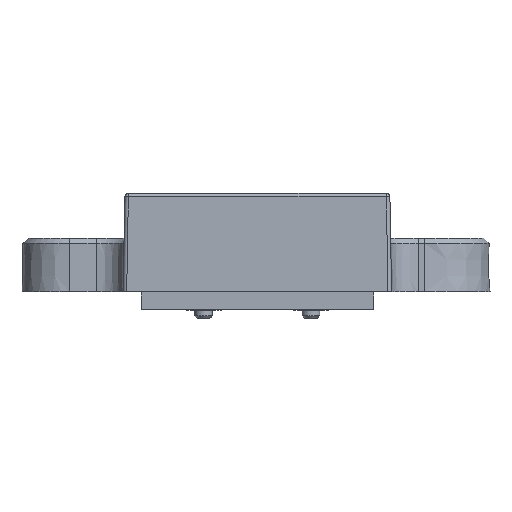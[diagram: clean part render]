
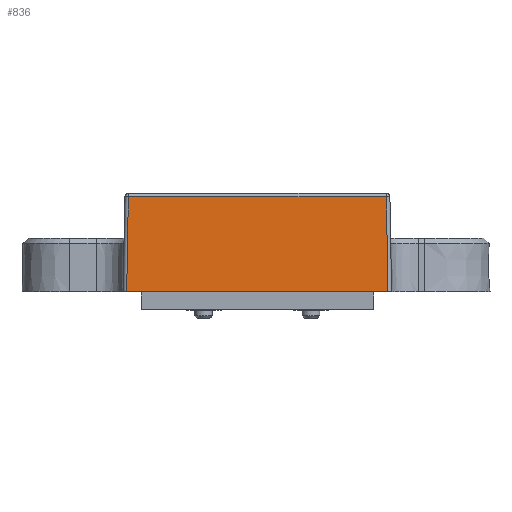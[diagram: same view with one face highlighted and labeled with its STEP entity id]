
A CAD part, left-side view. The second image highlights one B-rep face of the part: STEP entity #836.
In plain terms, the highlighted planar face has unit normal (-1, 0, 0.018).
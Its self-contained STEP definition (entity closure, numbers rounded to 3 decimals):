
#836 = ADVANCED_FACE ( 'NONE', ( #12670 ), #2323, .F. ) ;
#1189 = DIRECTION ( 'NONE',  ( 0., -1., 0. ) ) ;
#1268 = EDGE_CURVE ( 'NONE', #3279, #5187, #12795, .T. ) ;
#1419 = CARTESIAN_POINT ( 'NONE',  ( -17., 7.3, -5.5 ) ) ;
#1677 = EDGE_CURVE ( 'NONE', #14530, #8210, #9608, .T. ) ;
#1957 = EDGE_CURVE ( 'NONE', #8210, #3279, #11774, .T. ) ;
#2185 = CARTESIAN_POINT ( 'NONE',  ( -16.907, -7.207, -0.197 ) ) ;
#2323 = PLANE ( 'NONE',  #6677 ) ;
#2453 = CARTESIAN_POINT ( 'NONE',  ( -17., -7.3, -5.5 ) ) ;
#3279 = VERTEX_POINT ( 'NONE', #13879 ) ;
#3854 = DIRECTION ( 'NONE',  ( -0.017, 0.017, -1. ) ) ;
#5187 = VERTEX_POINT ( 'NONE', #9786 ) ;
#5796 = CARTESIAN_POINT ( 'NONE',  ( -16.907, 7.207, -0.197 ) ) ;
#6032 = DIRECTION ( 'NONE',  ( 0., -1., 0. ) ) ;
#6677 = AXIS2_PLACEMENT_3D ( 'NONE', #6950, #11542, #1189 ) ;
#6803 = DIRECTION ( 'NONE',  ( 0., 1., 0. ) ) ;
#6950 = CARTESIAN_POINT ( 'NONE',  ( -16.954, 0., -2.848 ) ) ;
#7079 = DIRECTION ( 'NONE',  ( 0.017, 0.017, 1. ) ) ;
#7343 = CARTESIAN_POINT ( 'NONE',  ( -17., 7.3, -5.5 ) ) ;
#8210 = VERTEX_POINT ( 'NONE', #7343 ) ;
#8333 = EDGE_CURVE ( 'NONE', #5187, #14530, #12531, .T. ) ;
#9608 = LINE ( 'NONE', #14212, #10751 ) ;
#9786 = CARTESIAN_POINT ( 'NONE',  ( -16.907, -7.207, -0.197 ) ) ;
#10751 = VECTOR ( 'NONE', #3854, 1000. ) ;
#11542 = DIRECTION ( 'NONE',  ( 1., 0., -0.017 ) ) ;
#11774 = LINE ( 'NONE', #1419, #14075 ) ;
#12416 = ORIENTED_EDGE ( 'NONE', *, *, #1957, .T. ) ;
#12531 = LINE ( 'NONE', #2185, #13412 ) ;
#12670 = FACE_OUTER_BOUND ( 'NONE', #13155, .T. ) ;
#12795 = LINE ( 'NONE', #2453, #13021 ) ;
#13021 = VECTOR ( 'NONE', #7079, 1000. ) ;
#13107 = ORIENTED_EDGE ( 'NONE', *, *, #8333, .T. ) ;
#13155 = EDGE_LOOP ( 'NONE', ( #13107, #14629, #12416, #13996 ) ) ;
#13412 = VECTOR ( 'NONE', #6803, 1000. ) ;
#13879 = CARTESIAN_POINT ( 'NONE',  ( -17., -7.3, -5.5 ) ) ;
#13996 = ORIENTED_EDGE ( 'NONE', *, *, #1268, .T. ) ;
#14075 = VECTOR ( 'NONE', #6032, 1000. ) ;
#14212 = CARTESIAN_POINT ( 'NONE',  ( -16.907, 7.207, -0.197 ) ) ;
#14530 = VERTEX_POINT ( 'NONE', #5796 ) ;
#14629 = ORIENTED_EDGE ( 'NONE', *, *, #1677, .T. ) ;
